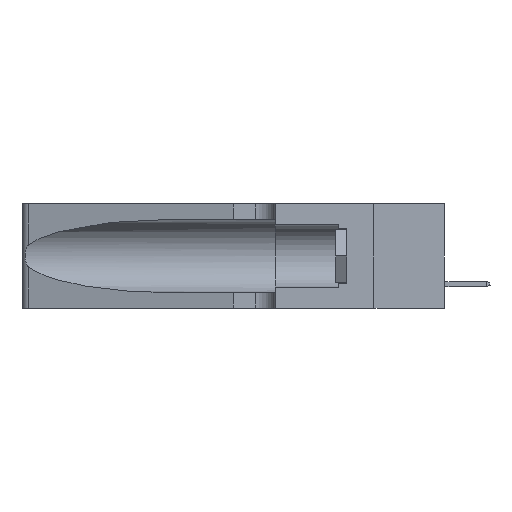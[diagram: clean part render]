
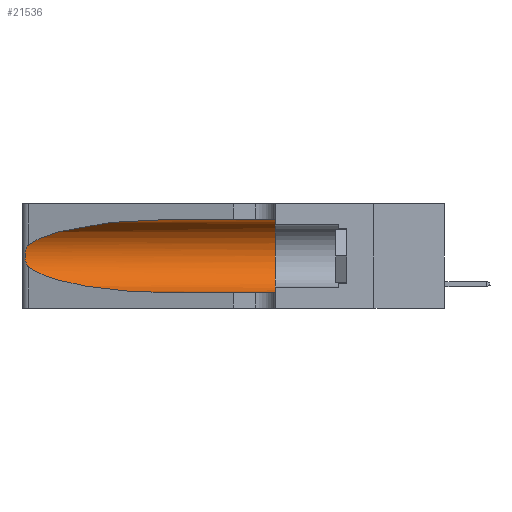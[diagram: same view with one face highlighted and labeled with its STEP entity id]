
A CAD part, left-side view. The second image highlights one B-rep face of the part: STEP entity #21536.
In plain terms, the highlighted cylindrical face has radius 3.308 mm (diameter 6.617 mm), a partial arc.
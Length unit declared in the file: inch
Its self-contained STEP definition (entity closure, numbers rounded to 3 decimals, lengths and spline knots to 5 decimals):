
#833 = CARTESIAN_POINT ( 'NONE',  ( 0.25555, 1.22993, 0.14849 ) ) ;
#1835 = VERTEX_POINT ( 'NONE', #19290 ) ;
#1912 = CYLINDRICAL_SURFACE ( 'NONE', #36071, 0.13025 ) ;
#5010 = CARTESIAN_POINT ( 'NONE',  ( 0.1305, 0.72297, 0.31525 ) ) ;
#5064 = DIRECTION ( 'NONE',  ( 0., -1., 0. ) ) ;
#5111 = EDGE_CURVE ( 'NONE', #1835, #33752, #15464, .T. ) ;
#5611 = CARTESIAN_POINT ( 'NONE',  ( 0.25487, 1.22718, 0.14631 ) ) ;
#6302 =( BOUNDED_CURVE ( )  B_SPLINE_CURVE ( 3, ( #5611, #32767, #12114, #18142 ),
 .UNSPECIFIED., .F., .F. ) 
 B_SPLINE_CURVE_WITH_KNOTS ( ( 4, 4 ),
 ( 3.44316, 4.71239 ),
 .UNSPECIFIED. ) 
 CURVE ( )  GEOMETRIC_REPRESENTATION_ITEM ( )  RATIONAL_B_SPLINE_CURVE ( ( 1., 0.87, 0.87, 1. ) ) 
 REPRESENTATION_ITEM ( '' )  );
#7241 = CARTESIAN_POINT ( 'NONE',  ( 0.25487, 1.22718, 0.22369 ) ) ;
#7752 = ORIENTED_EDGE ( 'NONE', *, *, #26958, .T. ) ;
#8469 = ORIENTED_EDGE ( 'NONE', *, *, #28606, .T. ) ;
#8561 =( BOUNDED_CURVE ( )  B_SPLINE_CURVE ( 3, ( #5010, #29147, #35152, #17083 ),
 .UNSPECIFIED., .F., .F. ) 
 B_SPLINE_CURVE_WITH_KNOTS ( ( 4, 4 ),
 ( 1.5708, 2.84003 ),
 .UNSPECIFIED. ) 
 CURVE ( )  GEOMETRIC_REPRESENTATION_ITEM ( )  RATIONAL_B_SPLINE_CURVE ( ( 1., 0.87, 0.87, 1. ) ) 
 REPRESENTATION_ITEM ( '' )  );
#8834 = CARTESIAN_POINT ( 'NONE',  ( 0.25856, 1.23593, 0.16098 ) ) ;
#8846 = VECTOR ( 'NONE', #16719, 39.37008 ) ;
#9126 = CARTESIAN_POINT ( 'NONE',  ( 0.25639, 1.23186, 0.15144 ) ) ;
#9769 = VECTOR ( 'NONE', #33787, 39.37008 ) ;
#10017 = CARTESIAN_POINT ( 'NONE',  ( 0.1305, 1.61858, 0.185 ) ) ;
#10731 = CARTESIAN_POINT ( 'NONE',  ( 0.1305, 0.72297, 0.31525 ) ) ;
#11780 = EDGE_LOOP ( 'NONE', ( #8469, #13433, #13724, #7752, #13667, #22770 ) ) ;
#12114 = CARTESIAN_POINT ( 'NONE',  ( 0.18966, 0.96281, 0.05475 ) ) ;
#12258 = CARTESIAN_POINT ( 'NONE',  ( 0.25789, 1.23486, 0.15765 ) ) ;
#13433 = ORIENTED_EDGE ( 'NONE', *, *, #5111, .T. ) ;
#13446 = CARTESIAN_POINT ( 'NONE',  ( 0.25639, 1.23184, 0.21858 ) ) ;
#13667 = ORIENTED_EDGE ( 'NONE', *, *, #38081, .F. ) ;
#13724 = ORIENTED_EDGE ( 'NONE', *, *, #22140, .T. ) ;
#15328 = LINE ( 'NONE', #37963, #8846 ) ;
#15464 = B_SPLINE_CURVE_WITH_KNOTS ( 'NONE', 3,
 ( #7241, #28100, #13446, #34398, #16452, #37424, #19459, #29056, #38725, #8834, #12258, #9126, #833, #18895 ),
 .UNSPECIFIED., .F., .F.,
 ( 4, 2, 2, 2, 2, 2, 4 ),
 ( 0., 0.00027, 0.00053, 0.00107, 0.0016, 0.00187, 0.00214 ),
 .UNSPECIFIED. ) ;
#16452 = CARTESIAN_POINT ( 'NONE',  ( 0.25854, 1.2359, 0.20912 ) ) ;
#16719 = DIRECTION ( 'NONE',  ( 0., -1., 0. ) ) ;
#17083 = CARTESIAN_POINT ( 'NONE',  ( 0.25487, 1.22718, 0.22369 ) ) ;
#18142 = CARTESIAN_POINT ( 'NONE',  ( 0.1305, 0.72297, 0.05475 ) ) ;
#18184 = VERTEX_POINT ( 'NONE', #30052 ) ;
#18895 = CARTESIAN_POINT ( 'NONE',  ( 0.25487, 1.22718, 0.14631 ) ) ;
#19290 = CARTESIAN_POINT ( 'NONE',  ( 0.25487, 1.22718, 0.22369 ) ) ;
#19459 = CARTESIAN_POINT ( 'NONE',  ( 0.26075, 1.23896, 0.19203 ) ) ;
#19729 = CARTESIAN_POINT ( 'NONE',  ( 0.1305, 0.35, 0.185 ) ) ;
#19735 = FACE_OUTER_BOUND ( 'NONE', #11780, .T. ) ;
#20242 = DIRECTION ( 'NONE',  ( 0., 0., 1. ) ) ;
#21536 = ADVANCED_FACE ( 'NONE', ( #19735 ), #1912, .F. ) ;
#22140 = EDGE_CURVE ( 'NONE', #33752, #35884, #6302, .T. ) ;
#22770 = ORIENTED_EDGE ( 'NONE', *, *, #26301, .F. ) ;
#22972 = AXIS2_PLACEMENT_3D ( 'NONE', #19729, #38222, #20242 ) ;
#23852 = LINE ( 'NONE', #28020, #9769 ) ;
#24392 = CARTESIAN_POINT ( 'NONE',  ( 0.1305, 0.35, 0.31525 ) ) ;
#26301 = EDGE_CURVE ( 'NONE', #30581, #28951, #23852, .T. ) ;
#26958 = EDGE_CURVE ( 'NONE', #35884, #18184, #15328, .T. ) ;
#28020 = CARTESIAN_POINT ( 'NONE',  ( 0.1305, 1.61858, 0.31525 ) ) ;
#28100 = CARTESIAN_POINT ( 'NONE',  ( 0.25555, 1.22994, 0.2215 ) ) ;
#28606 = EDGE_CURVE ( 'NONE', #30581, #1835, #8561, .T. ) ;
#28806 = DIRECTION ( 'NONE',  ( 0., 0., -1. ) ) ;
#28951 = VERTEX_POINT ( 'NONE', #24392 ) ;
#29056 = CARTESIAN_POINT ( 'NONE',  ( 0.26075, 1.23896, 0.178 ) ) ;
#29147 = CARTESIAN_POINT ( 'NONE',  ( 0.18966, 0.96281, 0.31525 ) ) ;
#30052 = CARTESIAN_POINT ( 'NONE',  ( 0.1305, 0.35, 0.05475 ) ) ;
#30085 = CARTESIAN_POINT ( 'NONE',  ( 0.25487, 1.22718, 0.14631 ) ) ;
#30581 = VERTEX_POINT ( 'NONE', #10731 ) ;
#31404 = CARTESIAN_POINT ( 'NONE',  ( 0.1305, 0.72297, 0.05475 ) ) ;
#31820 = CIRCLE ( 'NONE', #22972, 0.13025 ) ;
#32767 = CARTESIAN_POINT ( 'NONE',  ( 0.2373, 1.15595, 0.08982 ) ) ;
#33752 = VERTEX_POINT ( 'NONE', #30085 ) ;
#33787 = DIRECTION ( 'NONE',  ( 0., -1., 0. ) ) ;
#34398 = CARTESIAN_POINT ( 'NONE',  ( 0.25787, 1.23484, 0.2124 ) ) ;
#35152 = CARTESIAN_POINT ( 'NONE',  ( 0.2373, 1.15595, 0.28018 ) ) ;
#35884 = VERTEX_POINT ( 'NONE', #31404 ) ;
#36071 = AXIS2_PLACEMENT_3D ( 'NONE', #10017, #5064, #28806 ) ;
#37424 = CARTESIAN_POINT ( 'NONE',  ( 0.26018, 1.23835, 0.19895 ) ) ;
#37963 = CARTESIAN_POINT ( 'NONE',  ( 0.1305, 1.61858, 0.05475 ) ) ;
#38081 = EDGE_CURVE ( 'NONE', #28951, #18184, #31820, .T. ) ;
#38222 = DIRECTION ( 'NONE',  ( 0., 1., 0. ) ) ;
#38725 = CARTESIAN_POINT ( 'NONE',  ( 0.26017, 1.23833, 0.17102 ) ) ;
